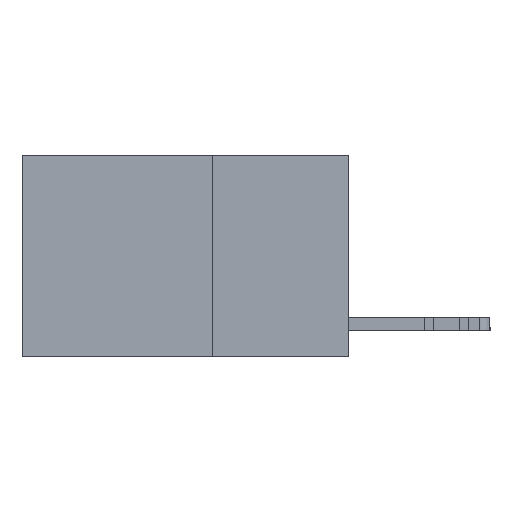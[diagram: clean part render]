
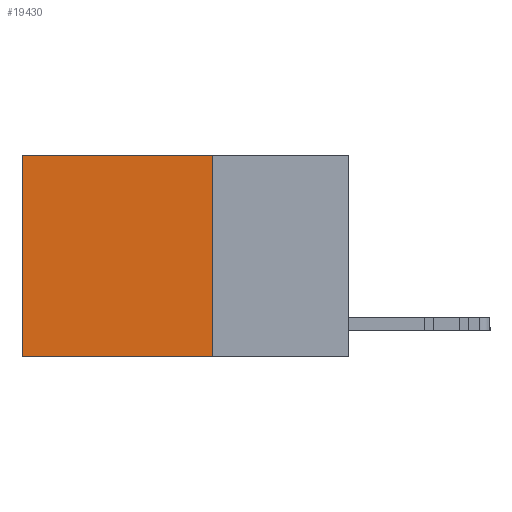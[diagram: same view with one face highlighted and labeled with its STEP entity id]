
A CAD part, left-side view. The second image highlights one B-rep face of the part: STEP entity #19430.
In plain terms, the highlighted planar face has unit normal (-1, 0, 0).
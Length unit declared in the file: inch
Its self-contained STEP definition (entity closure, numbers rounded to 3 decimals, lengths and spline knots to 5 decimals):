
#610 = DIRECTION ( 'NONE',  ( 0., 0., -1. ) ) ;
#734 = CARTESIAN_POINT ( 'NONE',  ( 0.2625, 0.6, 0. ) ) ;
#849 = DIRECTION ( 'NONE',  ( 0., 1., 0. ) ) ;
#1834 = VECTOR ( 'NONE', #610, 39.37008 ) ;
#3110 = LINE ( 'NONE', #19136, #9057 ) ;
#3950 = EDGE_CURVE ( 'NONE', #20255, #21081, #21873, .T. ) ;
#5271 = ORIENTED_EDGE ( 'NONE', *, *, #29245, .F. ) ;
#6052 = PLANE ( 'NONE',  #7410 ) ;
#7410 = AXIS2_PLACEMENT_3D ( 'NONE', #15281, #12718, #19956 ) ;
#7653 = DIRECTION ( 'NONE',  ( 0., 1., 0. ) ) ;
#9057 = VECTOR ( 'NONE', #7653, 39.37008 ) ;
#9518 = CARTESIAN_POINT ( 'NONE',  ( 0.2625, 0.25, -0.37 ) ) ;
#9781 = VERTEX_POINT ( 'NONE', #20396 ) ;
#10673 = VECTOR ( 'NONE', #28578, 39.37008 ) ;
#11719 = ORIENTED_EDGE ( 'NONE', *, *, #14547, .F. ) ;
#12718 = DIRECTION ( 'NONE',  ( 1., 0., 0. ) ) ;
#14105 = VECTOR ( 'NONE', #849, 39.37008 ) ;
#14547 = EDGE_CURVE ( 'NONE', #20255, #18502, #14827, .T. ) ;
#14827 = LINE ( 'NONE', #21486, #1834 ) ;
#15281 = CARTESIAN_POINT ( 'NONE',  ( 0.2625, 0.25, 0. ) ) ;
#17399 = FACE_OUTER_BOUND ( 'NONE', #22914, .T. ) ;
#17593 = EDGE_CURVE ( 'NONE', #21081, #9781, #28428, .T. ) ;
#18502 = VERTEX_POINT ( 'NONE', #9518 ) ;
#19136 = CARTESIAN_POINT ( 'NONE',  ( 0.2625, 0.25, -0.37 ) ) ;
#19162 = ORIENTED_EDGE ( 'NONE', *, *, #3950, .T. ) ;
#19430 = ADVANCED_FACE ( 'NONE', ( #17399 ), #6052, .F. ) ;
#19956 = DIRECTION ( 'NONE',  ( 0., 0., -1. ) ) ;
#20255 = VERTEX_POINT ( 'NONE', #23383 ) ;
#20396 = CARTESIAN_POINT ( 'NONE',  ( 0.2625, 0.6, -0.37 ) ) ;
#21081 = VERTEX_POINT ( 'NONE', #734 ) ;
#21486 = CARTESIAN_POINT ( 'NONE',  ( 0.2625, 0.25, 0. ) ) ;
#21873 = LINE ( 'NONE', #24420, #14105 ) ;
#22914 = EDGE_LOOP ( 'NONE', ( #27816, #5271, #11719, #19162 ) ) ;
#23383 = CARTESIAN_POINT ( 'NONE',  ( 0.2625, 0.25, 0. ) ) ;
#24420 = CARTESIAN_POINT ( 'NONE',  ( 0.2625, 0.25, 0. ) ) ;
#26314 = CARTESIAN_POINT ( 'NONE',  ( 0.2625, 0.6, 0. ) ) ;
#27816 = ORIENTED_EDGE ( 'NONE', *, *, #17593, .T. ) ;
#28428 = LINE ( 'NONE', #26314, #10673 ) ;
#28578 = DIRECTION ( 'NONE',  ( 0., 0., -1. ) ) ;
#29245 = EDGE_CURVE ( 'NONE', #18502, #9781, #3110, .T. ) ;
